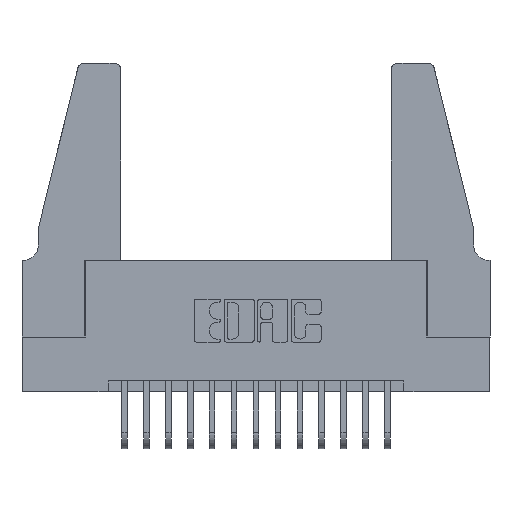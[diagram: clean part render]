
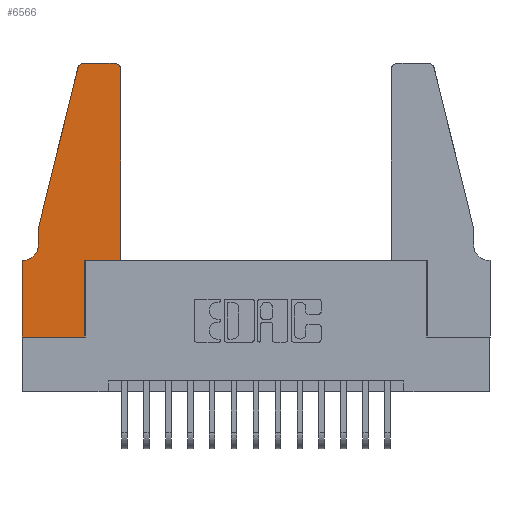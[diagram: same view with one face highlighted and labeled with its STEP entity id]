
A CAD part, top view. The second image highlights one B-rep face of the part: STEP entity #6566.
In plain terms, the highlighted planar face has unit normal (0, 0, 1).
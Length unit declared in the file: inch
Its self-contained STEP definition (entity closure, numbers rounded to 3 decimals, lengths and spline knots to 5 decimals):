
#135 = ORIENTED_EDGE ( 'NONE', *, *, #12101, .T. ) ;
#368 = VERTEX_POINT ( 'NONE', #7649 ) ;
#653 = EDGE_CURVE ( 'NONE', #5780, #1830, #6383, .T. ) ;
#714 = DIRECTION ( 'NONE',  ( 1., 0., 0. ) ) ;
#730 = DIRECTION ( 'NONE',  ( 1., 0., 0. ) ) ;
#818 = ORIENTED_EDGE ( 'NONE', *, *, #653, .T. ) ;
#1039 = EDGE_CURVE ( 'NONE', #3630, #13521, #7135, .T. ) ;
#1115 = AXIS2_PLACEMENT_3D ( 'NONE', #1941, #10547, #3223 ) ;
#1169 = CARTESIAN_POINT ( 'NONE',  ( 0.284, 1.22, 0.37 ) ) ;
#1194 = CARTESIAN_POINT ( 'NONE',  ( 0., 0., 0.37 ) ) ;
#1307 = CARTESIAN_POINT ( 'NONE',  ( 0.2865, 0.35, 0.37 ) ) ;
#1495 = CARTESIAN_POINT ( 'NONE',  ( 0.0055, 0.35, 0.37 ) ) ;
#1667 = CARTESIAN_POINT ( 'NONE',  ( 0., 0.35, 0.37 ) ) ;
#1830 = VERTEX_POINT ( 'NONE', #7924 ) ;
#1941 = CARTESIAN_POINT ( 'NONE',  ( 0.4205, 1.22, 0.37 ) ) ;
#2458 = DIRECTION ( 'NONE',  ( 1., 0., 0. ) ) ;
#2514 = VECTOR ( 'NONE', #10595, 39.37008 ) ;
#2721 = CARTESIAN_POINT ( 'NONE',  ( 0.2865, 0.35, 0.37 ) ) ;
#2921 = CARTESIAN_POINT ( 'NONE',  ( 0.0055, 0.42, 0.37 ) ) ;
#3149 = VECTOR ( 'NONE', #714, 39.37008 ) ;
#3204 = VERTEX_POINT ( 'NONE', #15566 ) ;
#3223 = DIRECTION ( 'NONE',  ( 1., 0., 0. ) ) ;
#3285 = CARTESIAN_POINT ( 'NONE',  ( 0.2605, 1.25, 0.37 ) ) ;
#3630 = VERTEX_POINT ( 'NONE', #1667 ) ;
#3652 = EDGE_CURVE ( 'NONE', #3204, #368, #3759, .T. ) ;
#3759 = LINE ( 'NONE', #11535, #9876 ) ;
#4155 = ORIENTED_EDGE ( 'NONE', *, *, #1039, .T. ) ;
#4178 = DIRECTION ( 'NONE',  ( -1., 0., 0. ) ) ;
#4200 = AXIS2_PLACEMENT_3D ( 'NONE', #2921, #11472, #4178 ) ;
#4334 = EDGE_CURVE ( 'NONE', #9853, #10650, #14544, .T. ) ;
#5153 = VERTEX_POINT ( 'NONE', #11824 ) ;
#5383 = CARTESIAN_POINT ( 'NONE',  ( 0., 0.35, 0.37 ) ) ;
#5416 = VECTOR ( 'NONE', #730, 39.37008 ) ;
#5420 = CARTESIAN_POINT ( 'NONE',  ( 0.0755, 0.35, 0.37 ) ) ;
#5595 = LINE ( 'NONE', #5420, #11690 ) ;
#5693 = CARTESIAN_POINT ( 'NONE',  ( 0.4505, 0.35, 0.37 ) ) ;
#5780 = VERTEX_POINT ( 'NONE', #6382 ) ;
#5787 = VERTEX_POINT ( 'NONE', #2721 ) ;
#5791 = LINE ( 'NONE', #3285, #2514 ) ;
#6217 = LINE ( 'NONE', #12589, #8695 ) ;
#6382 = CARTESIAN_POINT ( 'NONE',  ( 0.25487, 1.22718, 0.37 ) ) ;
#6383 = LINE ( 'NONE', #11154, #12473 ) ;
#6430 = LINE ( 'NONE', #5693, #3149 ) ;
#6474 = CIRCLE ( 'NONE', #1115, 0.03 ) ;
#6566 = ADVANCED_FACE ( 'NONE', ( #10842 ), #10251, .T. ) ;
#6610 = DIRECTION ( 'NONE',  ( 1., 0., 0. ) ) ;
#6660 = DIRECTION ( 'NONE',  ( -1., 0., 0. ) ) ;
#7135 = LINE ( 'NONE', #15453, #13251 ) ;
#7226 = EDGE_LOOP ( 'NONE', ( #8409, #135, #818, #9651, #7504, #14906, #4155, #11739, #15527, #15061, #7982, #14990 ) ) ;
#7263 = CARTESIAN_POINT ( 'NONE',  ( 0.4205, 1.25, 0.37 ) ) ;
#7366 = VECTOR ( 'NONE', #12381, 39.37008 ) ;
#7504 = ORIENTED_EDGE ( 'NONE', *, *, #4334, .T. ) ;
#7649 = CARTESIAN_POINT ( 'NONE',  ( 0.4505, 1.22, 0.37 ) ) ;
#7924 = CARTESIAN_POINT ( 'NONE',  ( 0.0755, 0.5, 0.37 ) ) ;
#7982 = ORIENTED_EDGE ( 'NONE', *, *, #3652, .T. ) ;
#8166 = CARTESIAN_POINT ( 'NONE',  ( 0., 0., 0.37 ) ) ;
#8175 = EDGE_CURVE ( 'NONE', #13521, #5153, #14773, .T. ) ;
#8409 = ORIENTED_EDGE ( 'NONE', *, *, #9029, .T. ) ;
#8503 = CARTESIAN_POINT ( 'NONE',  ( 0.284, 1.25, 0.37 ) ) ;
#8695 = VECTOR ( 'NONE', #8913, 39.37008 ) ;
#8844 = EDGE_CURVE ( 'NONE', #10650, #3630, #5595, .T. ) ;
#8867 = DIRECTION ( 'NONE',  ( -0.239, -0.971, 0. ) ) ;
#8913 = DIRECTION ( 'NONE',  ( 0., -1., 0. ) ) ;
#9029 = EDGE_CURVE ( 'NONE', #10418, #15715, #5791, .T. ) ;
#9651 = ORIENTED_EDGE ( 'NONE', *, *, #15934, .T. ) ;
#9802 = DIRECTION ( 'NONE',  ( 0., 0., 1. ) ) ;
#9838 = CARTESIAN_POINT ( 'NONE',  ( 0.0755, 0.42, 0.37 ) ) ;
#9853 = VERTEX_POINT ( 'NONE', #9838 ) ;
#9876 = VECTOR ( 'NONE', #10334, 39.37008 ) ;
#10186 = DIRECTION ( 'NONE',  ( 0., -1., 0. ) ) ;
#10251 = PLANE ( 'NONE',  #15139 ) ;
#10334 = DIRECTION ( 'NONE',  ( 0., 1., 0. ) ) ;
#10418 = VERTEX_POINT ( 'NONE', #7263 ) ;
#10547 = DIRECTION ( 'NONE',  ( 0., 0., 1. ) ) ;
#10595 = DIRECTION ( 'NONE',  ( -1., 0., 0. ) ) ;
#10650 = VERTEX_POINT ( 'NONE', #1495 ) ;
#10842 = FACE_OUTER_BOUND ( 'NONE', #7226, .T. ) ;
#11154 = CARTESIAN_POINT ( 'NONE',  ( 0.0755, 0.5, 0.37 ) ) ;
#11351 = LINE ( 'NONE', #1307, #7366 ) ;
#11472 = DIRECTION ( 'NONE',  ( 0., 0., -1. ) ) ;
#11535 = CARTESIAN_POINT ( 'NONE',  ( 0.4505, 0.35, 0.37 ) ) ;
#11690 = VECTOR ( 'NONE', #6660, 39.37008 ) ;
#11739 = ORIENTED_EDGE ( 'NONE', *, *, #8175, .T. ) ;
#11818 = EDGE_CURVE ( 'NONE', #368, #10418, #6474, .T. ) ;
#11824 = CARTESIAN_POINT ( 'NONE',  ( 0.2865, 0., 0.37 ) ) ;
#11984 = CIRCLE ( 'NONE', #14276, 0.03 ) ;
#12101 = EDGE_CURVE ( 'NONE', #15715, #5780, #11984, .T. ) ;
#12381 = DIRECTION ( 'NONE',  ( 0., 1., 0. ) ) ;
#12473 = VECTOR ( 'NONE', #8867, 39.37008 ) ;
#12589 = CARTESIAN_POINT ( 'NONE',  ( 0.0755, 0.5, 0.37 ) ) ;
#13251 = VECTOR ( 'NONE', #10186, 39.37008 ) ;
#13521 = VERTEX_POINT ( 'NONE', #1194 ) ;
#13925 = DIRECTION ( 'NONE',  ( 0., 0., 1. ) ) ;
#14276 = AXIS2_PLACEMENT_3D ( 'NONE', #1169, #9802, #2458 ) ;
#14544 = CIRCLE ( 'NONE', #4200, 0.07 ) ;
#14773 = LINE ( 'NONE', #8166, #5416 ) ;
#14906 = ORIENTED_EDGE ( 'NONE', *, *, #8844, .T. ) ;
#14990 = ORIENTED_EDGE ( 'NONE', *, *, #11818, .T. ) ;
#15061 = ORIENTED_EDGE ( 'NONE', *, *, #15266, .T. ) ;
#15139 = AXIS2_PLACEMENT_3D ( 'NONE', #5383, #13925, #6610 ) ;
#15266 = EDGE_CURVE ( 'NONE', #5787, #3204, #6430, .T. ) ;
#15453 = CARTESIAN_POINT ( 'NONE',  ( 0., 0., 0.37 ) ) ;
#15527 = ORIENTED_EDGE ( 'NONE', *, *, #15853, .T. ) ;
#15566 = CARTESIAN_POINT ( 'NONE',  ( 0.4505, 0.35, 0.37 ) ) ;
#15715 = VERTEX_POINT ( 'NONE', #8503 ) ;
#15853 = EDGE_CURVE ( 'NONE', #5153, #5787, #11351, .T. ) ;
#15934 = EDGE_CURVE ( 'NONE', #1830, #9853, #6217, .T. ) ;
